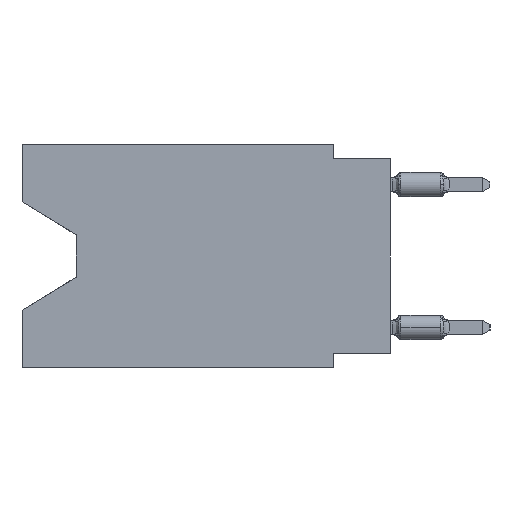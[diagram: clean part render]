
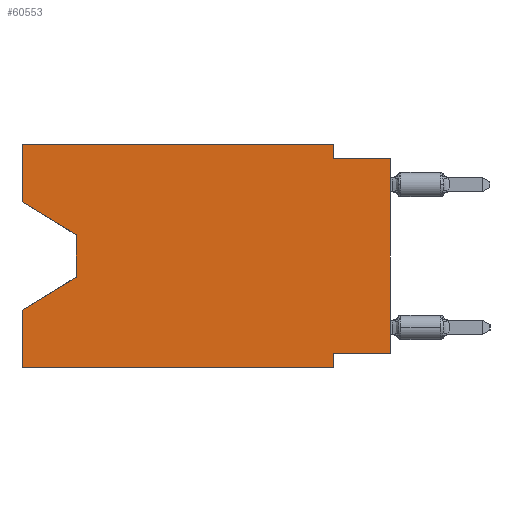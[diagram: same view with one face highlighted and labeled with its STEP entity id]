
A CAD part, left-side view. The second image highlights one B-rep face of the part: STEP entity #60553.
In plain terms, the highlighted planar face has unit normal (-1, 0, 0).
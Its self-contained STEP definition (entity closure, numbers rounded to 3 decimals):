
#1152 = LINE ( 'NONE', #20269, #17143 ) ;
#2500 = ORIENTED_EDGE ( 'NONE', *, *, #44927, .T. ) ;
#3782 = CARTESIAN_POINT ( 'NONE',  ( 0., 0., -0.635 ) ) ;
#4029 = CARTESIAN_POINT ( 'NONE',  ( 0., 16.383, -7.36 ) ) ;
#5582 = DIRECTION ( 'NONE',  ( 0., 0., 1. ) ) ;
#6589 = ORIENTED_EDGE ( 'NONE', *, *, #53849, .T. ) ;
#6876 = DIRECTION ( 'NONE',  ( 0., -1., 0. ) ) ;
#7255 = CARTESIAN_POINT ( 'NONE',  ( 0., 2.54, -9.271 ) ) ;
#7753 = VERTEX_POINT ( 'NONE', #3782 ) ;
#8658 = LINE ( 'NONE', #17430, #60107 ) ;
#8998 = CARTESIAN_POINT ( 'NONE',  ( 0., 16.383, 0. ) ) ;
#9912 = DIRECTION ( 'NONE',  ( 0., 0., 1. ) ) ;
#10658 = VERTEX_POINT ( 'NONE', #13229 ) ;
#11497 = VERTEX_POINT ( 'NONE', #23878 ) ;
#11499 = CARTESIAN_POINT ( 'NONE',  ( 0., 16.383, -9.906 ) ) ;
#11845 = VECTOR ( 'NONE', #6876, 1000. ) ;
#12731 = DIRECTION ( 'NONE',  ( 0., -0.855, -0.519 ) ) ;
#13084 = VECTOR ( 'NONE', #22665, 1000. ) ;
#13229 = CARTESIAN_POINT ( 'NONE',  ( 0., 2.54, -9.906 ) ) ;
#15328 = CARTESIAN_POINT ( 'NONE',  ( 0., 16.383, -2.546 ) ) ;
#15783 = LINE ( 'NONE', #19545, #28578 ) ;
#16304 = CARTESIAN_POINT ( 'NONE',  ( 0., 16.383, 0. ) ) ;
#16950 = VECTOR ( 'NONE', #34364, 1000. ) ;
#17143 = VECTOR ( 'NONE', #44764, 1000. ) ;
#17430 = CARTESIAN_POINT ( 'NONE',  ( 0., 16.383, -2.546 ) ) ;
#18817 = EDGE_CURVE ( 'NONE', #37958, #10658, #37845, .T. ) ;
#19545 = CARTESIAN_POINT ( 'NONE',  ( 0., 0., -0.635 ) ) ;
#19801 = EDGE_CURVE ( 'NONE', #50380, #44459, #8658, .T. ) ;
#20269 = CARTESIAN_POINT ( 'NONE',  ( 0., 2.54, -9.906 ) ) ;
#21374 = AXIS2_PLACEMENT_3D ( 'NONE', #16304, #58698, #54298 ) ;
#22197 = DIRECTION ( 'NONE',  ( 0., 0., -1. ) ) ;
#22297 = ORIENTED_EDGE ( 'NONE', *, *, #19801, .T. ) ;
#22665 = DIRECTION ( 'NONE',  ( 0., 0., 1. ) ) ;
#23340 = VERTEX_POINT ( 'NONE', #4029 ) ;
#23878 = CARTESIAN_POINT ( 'NONE',  ( 0., 0., -9.271 ) ) ;
#24774 = ORIENTED_EDGE ( 'NONE', *, *, #18817, .T. ) ;
#26564 = EDGE_LOOP ( 'NONE', ( #22297, #6589, #2500, #39828, #24774, #61763, #57051, #29102, #60302, #40150, #61910, #58369 ) ) ;
#26591 = LINE ( 'NONE', #40116, #34508 ) ;
#26724 = VERTEX_POINT ( 'NONE', #8998 ) ;
#26803 = EDGE_CURVE ( 'NONE', #50380, #26724, #47588, .T. ) ;
#27479 = VECTOR ( 'NONE', #42093, 1000. ) ;
#28578 = VECTOR ( 'NONE', #53154, 1000. ) ;
#29102 = ORIENTED_EDGE ( 'NONE', *, *, #55732, .T. ) ;
#29214 = CARTESIAN_POINT ( 'NONE',  ( 0., 13.97, -4.013 ) ) ;
#30309 = EDGE_CURVE ( 'NONE', #37958, #23340, #43547, .T. ) ;
#31901 = EDGE_CURVE ( 'NONE', #61090, #7753, #15783, .T. ) ;
#33130 = CARTESIAN_POINT ( 'NONE',  ( 0., 16.383, -9.906 ) ) ;
#34086 = EDGE_CURVE ( 'NONE', #26724, #46126, #40443, .T. ) ;
#34155 = LINE ( 'NONE', #58337, #57794 ) ;
#34364 = DIRECTION ( 'NONE',  ( 0., -1., 0. ) ) ;
#34508 = VECTOR ( 'NONE', #22197, 1000. ) ;
#35451 = FACE_OUTER_BOUND ( 'NONE', #26564, .T. ) ;
#35729 = VERTEX_POINT ( 'NONE', #7255 ) ;
#36683 = LINE ( 'NONE', #59915, #53255 ) ;
#37432 = EDGE_CURVE ( 'NONE', #46126, #61090, #36683, .T. ) ;
#37845 = LINE ( 'NONE', #33130, #16950 ) ;
#37958 = VERTEX_POINT ( 'NONE', #11499 ) ;
#38524 = CARTESIAN_POINT ( 'NONE',  ( 0., 16.383, 0. ) ) ;
#38645 = VECTOR ( 'NONE', #9912, 1000. ) ;
#39828 = ORIENTED_EDGE ( 'NONE', *, *, #30309, .F. ) ;
#40116 = CARTESIAN_POINT ( 'NONE',  ( 0., 13.97, -4.013 ) ) ;
#40150 = ORIENTED_EDGE ( 'NONE', *, *, #37432, .F. ) ;
#40443 = LINE ( 'NONE', #55192, #11845 ) ;
#41347 = EDGE_CURVE ( 'NONE', #11497, #35729, #46485, .T. ) ;
#42093 = DIRECTION ( 'NONE',  ( 0., 1., 0. ) ) ;
#43547 = LINE ( 'NONE', #38524, #59704 ) ;
#43796 = CARTESIAN_POINT ( 'NONE',  ( 0., 16.383, 0. ) ) ;
#44459 = VERTEX_POINT ( 'NONE', #29214 ) ;
#44764 = DIRECTION ( 'NONE',  ( 0., 0., -1. ) ) ;
#44927 = EDGE_CURVE ( 'NONE', #59166, #23340, #34155, .T. ) ;
#46126 = VERTEX_POINT ( 'NONE', #61816 ) ;
#46485 = LINE ( 'NONE', #51499, #27479 ) ;
#46509 = CARTESIAN_POINT ( 'NONE',  ( 0., 13.97, -5.893 ) ) ;
#46843 = LINE ( 'NONE', #51552, #13084 ) ;
#47588 = LINE ( 'NONE', #43796, #38645 ) ;
#50380 = VERTEX_POINT ( 'NONE', #15328 ) ;
#51499 = CARTESIAN_POINT ( 'NONE',  ( 0., 0., -9.271 ) ) ;
#51552 = CARTESIAN_POINT ( 'NONE',  ( 0., 0., 0. ) ) ;
#53154 = DIRECTION ( 'NONE',  ( 0., -1., 0. ) ) ;
#53255 = VECTOR ( 'NONE', #55513, 1000. ) ;
#53849 = EDGE_CURVE ( 'NONE', #44459, #59166, #26591, .T. ) ;
#54298 = DIRECTION ( 'NONE',  ( 0., 0., -1. ) ) ;
#54603 = PLANE ( 'NONE',  #21374 ) ;
#55192 = CARTESIAN_POINT ( 'NONE',  ( 0., 16.383, 0. ) ) ;
#55513 = DIRECTION ( 'NONE',  ( 0., 0., -1. ) ) ;
#55732 = EDGE_CURVE ( 'NONE', #11497, #7753, #46843, .T. ) ;
#57051 = ORIENTED_EDGE ( 'NONE', *, *, #41347, .F. ) ;
#57794 = VECTOR ( 'NONE', #58957, 1000. ) ;
#58087 = EDGE_CURVE ( 'NONE', #35729, #10658, #1152, .T. ) ;
#58337 = CARTESIAN_POINT ( 'NONE',  ( 0., 13.97, -5.893 ) ) ;
#58369 = ORIENTED_EDGE ( 'NONE', *, *, #26803, .F. ) ;
#58698 = DIRECTION ( 'NONE',  ( 1., 0., 0. ) ) ;
#58957 = DIRECTION ( 'NONE',  ( 0., 0.855, -0.519 ) ) ;
#59166 = VERTEX_POINT ( 'NONE', #46509 ) ;
#59248 = CARTESIAN_POINT ( 'NONE',  ( 0., 2.54, -0.635 ) ) ;
#59704 = VECTOR ( 'NONE', #5582, 1000. ) ;
#59915 = CARTESIAN_POINT ( 'NONE',  ( 0., 2.54, 0. ) ) ;
#60107 = VECTOR ( 'NONE', #12731, 1000. ) ;
#60302 = ORIENTED_EDGE ( 'NONE', *, *, #31901, .F. ) ;
#60553 = ADVANCED_FACE ( 'NONE', ( #35451 ), #54603, .F. ) ;
#61090 = VERTEX_POINT ( 'NONE', #59248 ) ;
#61763 = ORIENTED_EDGE ( 'NONE', *, *, #58087, .F. ) ;
#61816 = CARTESIAN_POINT ( 'NONE',  ( 0., 2.54, 0. ) ) ;
#61910 = ORIENTED_EDGE ( 'NONE', *, *, #34086, .F. ) ;
